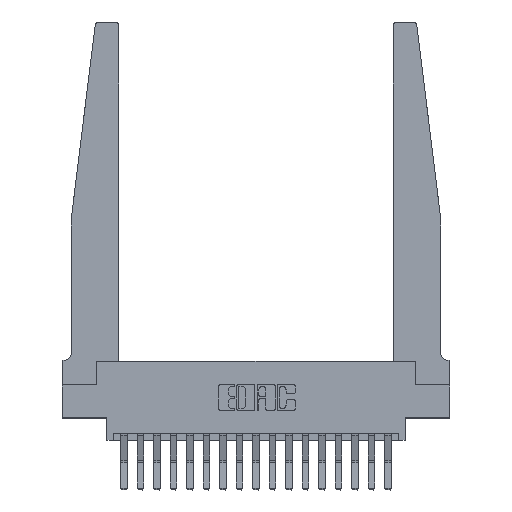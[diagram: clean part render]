
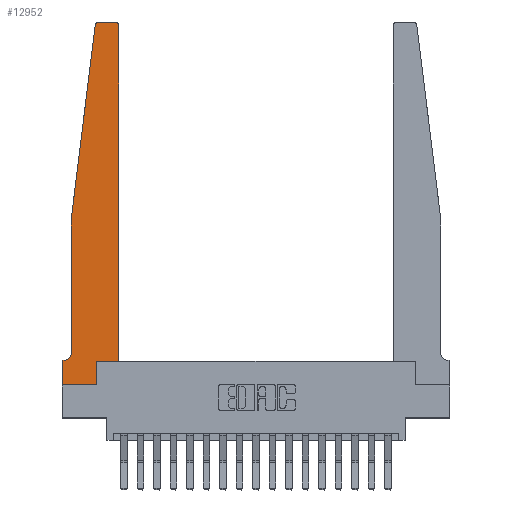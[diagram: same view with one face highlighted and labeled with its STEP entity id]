
A CAD part, top view. The second image highlights one B-rep face of the part: STEP entity #12952.
In plain terms, the highlighted planar face has unit normal (0, 0, 1).
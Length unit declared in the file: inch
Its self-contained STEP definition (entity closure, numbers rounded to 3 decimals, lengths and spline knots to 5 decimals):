
#132 = CARTESIAN_POINT ( 'NONE',  ( 0., 0.1875, 0.37 ) ) ;
#363 = VECTOR ( 'NONE', #8757, 39.37008 ) ;
#395 = VECTOR ( 'NONE', #5846, 39.37008 ) ;
#454 = CARTESIAN_POINT ( 'NONE',  ( 0.2605, 0., 0.37 ) ) ;
#477 = PLANE ( 'NONE',  #17138 ) ;
#569 = CARTESIAN_POINT ( 'NONE',  ( 0.24675, 2.72367, 0.37 ) ) ;
#772 = EDGE_CURVE ( 'NONE', #9024, #2285, #6179, .T. ) ;
#812 = ORIENTED_EDGE ( 'NONE', *, *, #9415, .T. ) ;
#907 = CARTESIAN_POINT ( 'NONE',  ( 0.395, 2.75, 0.37 ) ) ;
#1017 = EDGE_CURVE ( 'NONE', #3345, #19873, #10927, .T. ) ;
#1134 = ORIENTED_EDGE ( 'NONE', *, *, #4378, .T. ) ;
#1855 = CIRCLE ( 'NONE', #8939, 0.03 ) ;
#1858 = CARTESIAN_POINT ( 'NONE',  ( 0., 0., 0.37 ) ) ;
#1948 = VECTOR ( 'NONE', #12959, 39.37008 ) ;
#2080 = ORIENTED_EDGE ( 'NONE', *, *, #12305, .T. ) ;
#2121 = DIRECTION ( 'NONE',  ( -1., 0., 0. ) ) ;
#2285 = VERTEX_POINT ( 'NONE', #8772 ) ;
#2333 = VECTOR ( 'NONE', #6653, 39.37008 ) ;
#2542 = CARTESIAN_POINT ( 'NONE',  ( 0.425, 0.18, 0.37 ) ) ;
#3279 = VERTEX_POINT ( 'NONE', #5874 ) ;
#3345 = VERTEX_POINT ( 'NONE', #907 ) ;
#3388 = CARTESIAN_POINT ( 'NONE',  ( 0.425, 0.18, 0.37 ) ) ;
#3625 = CARTESIAN_POINT ( 'NONE',  ( 0.015, 0.2375, 0.37 ) ) ;
#3632 = EDGE_CURVE ( 'NONE', #3279, #8350, #10799, .T. ) ;
#3670 = LINE ( 'NONE', #9833, #16539 ) ;
#3738 = CIRCLE ( 'NONE', #11496, 0.03 ) ;
#3745 = VERTEX_POINT ( 'NONE', #15587 ) ;
#3759 = DIRECTION ( 'NONE',  ( -0.122, -0.992, 0. ) ) ;
#3786 = CARTESIAN_POINT ( 'NONE',  ( 0.27653, 2.72, 0.37 ) ) ;
#3845 = EDGE_CURVE ( 'NONE', #19873, #18053, #3738, .T. ) ;
#4378 = EDGE_CURVE ( 'NONE', #2285, #3745, #19816, .T. ) ;
#4546 = ORIENTED_EDGE ( 'NONE', *, *, #14837, .T. ) ;
#4710 = DIRECTION ( 'NONE',  ( 0., 0., 1. ) ) ;
#5146 = EDGE_CURVE ( 'NONE', #10796, #3345, #1855, .T. ) ;
#5281 = CARTESIAN_POINT ( 'NONE',  ( 0.395, 2.72, 0.37 ) ) ;
#5485 = DIRECTION ( 'NONE',  ( 1., 0., 0. ) ) ;
#5495 = CARTESIAN_POINT ( 'NONE',  ( 0.425, 2.72, 0.37 ) ) ;
#5846 = DIRECTION ( 'NONE',  ( 0., 1., 0. ) ) ;
#5874 = CARTESIAN_POINT ( 'NONE',  ( 0., 0., 0.37 ) ) ;
#5977 = DIRECTION ( 'NONE',  ( 0., -1., 0. ) ) ;
#6179 = LINE ( 'NONE', #16731, #19695 ) ;
#6653 = DIRECTION ( 'NONE',  ( -1., 0., 0. ) ) ;
#7195 = CARTESIAN_POINT ( 'NONE',  ( 0.27653, 2.75, 0.37 ) ) ;
#7223 = VECTOR ( 'NONE', #8010, 39.37008 ) ;
#8010 = DIRECTION ( 'NONE',  ( 0., -1., 0. ) ) ;
#8079 = DIRECTION ( 'NONE',  ( -1., 0., 0. ) ) ;
#8350 = VERTEX_POINT ( 'NONE', #454 ) ;
#8459 = EDGE_CURVE ( 'NONE', #11095, #10796, #19153, .T. ) ;
#8757 = DIRECTION ( 'NONE',  ( 1., 0., 0. ) ) ;
#8772 = CARTESIAN_POINT ( 'NONE',  ( 0.065, 0.2375, 0.37 ) ) ;
#8789 = VERTEX_POINT ( 'NONE', #132 ) ;
#8939 = AXIS2_PLACEMENT_3D ( 'NONE', #5281, #14077, #11458 ) ;
#8941 = VECTOR ( 'NONE', #19797, 39.37008 ) ;
#8980 = CARTESIAN_POINT ( 'NONE',  ( 0.065, 1.25, 0.37 ) ) ;
#9024 = VERTEX_POINT ( 'NONE', #8980 ) ;
#9089 = LINE ( 'NONE', #18223, #395 ) ;
#9396 = ORIENTED_EDGE ( 'NONE', *, *, #3632, .T. ) ;
#9415 = EDGE_CURVE ( 'NONE', #10102, #11095, #18305, .T. ) ;
#9480 = CARTESIAN_POINT ( 'NONE',  ( 0.065, 0.1875, 0.37 ) ) ;
#9833 = CARTESIAN_POINT ( 'NONE',  ( 0.065, 1.25, 0.37 ) ) ;
#10102 = VERTEX_POINT ( 'NONE', #13637 ) ;
#10314 = ORIENTED_EDGE ( 'NONE', *, *, #1017, .T. ) ;
#10402 = ORIENTED_EDGE ( 'NONE', *, *, #14713, .T. ) ;
#10688 = CARTESIAN_POINT ( 'NONE',  ( 0., 0., 0.37 ) ) ;
#10699 = CARTESIAN_POINT ( 'NONE',  ( 0.425, 0.18, 0.37 ) ) ;
#10796 = VERTEX_POINT ( 'NONE', #5495 ) ;
#10799 = LINE ( 'NONE', #10688, #8941 ) ;
#10888 = FACE_OUTER_BOUND ( 'NONE', #17705, .T. ) ;
#10927 = LINE ( 'NONE', #17325, #15064 ) ;
#11095 = VERTEX_POINT ( 'NONE', #3388 ) ;
#11170 = ORIENTED_EDGE ( 'NONE', *, *, #5146, .T. ) ;
#11389 = DIRECTION ( 'NONE',  ( 0., 0., 1. ) ) ;
#11458 = DIRECTION ( 'NONE',  ( 1., 0., 0. ) ) ;
#11496 = AXIS2_PLACEMENT_3D ( 'NONE', #3786, #11389, #5485 ) ;
#11811 = AXIS2_PLACEMENT_3D ( 'NONE', #3625, #15915, #2121 ) ;
#12305 = EDGE_CURVE ( 'NONE', #8350, #10102, #9089, .T. ) ;
#12462 = EDGE_CURVE ( 'NONE', #3745, #8789, #12516, .T. ) ;
#12516 = LINE ( 'NONE', #9480, #2333 ) ;
#12952 = ADVANCED_FACE ( 'NONE', ( #10888 ), #477, .T. ) ;
#12959 = DIRECTION ( 'NONE',  ( 0., 1., 0. ) ) ;
#13637 = CARTESIAN_POINT ( 'NONE',  ( 0.2605, 0.18, 0.37 ) ) ;
#14077 = DIRECTION ( 'NONE',  ( 0., 0., 1. ) ) ;
#14340 = ORIENTED_EDGE ( 'NONE', *, *, #8459, .T. ) ;
#14713 = EDGE_CURVE ( 'NONE', #8789, #3279, #18673, .T. ) ;
#14837 = EDGE_CURVE ( 'NONE', #18053, #9024, #3670, .T. ) ;
#15064 = VECTOR ( 'NONE', #8079, 39.37008 ) ;
#15121 = ORIENTED_EDGE ( 'NONE', *, *, #12462, .T. ) ;
#15587 = CARTESIAN_POINT ( 'NONE',  ( 0.015, 0.1875, 0.37 ) ) ;
#15788 = DIRECTION ( 'NONE',  ( 1., 0., 0. ) ) ;
#15915 = DIRECTION ( 'NONE',  ( 0., 0., -1. ) ) ;
#16340 = ORIENTED_EDGE ( 'NONE', *, *, #772, .T. ) ;
#16539 = VECTOR ( 'NONE', #3759, 39.37008 ) ;
#16636 = ORIENTED_EDGE ( 'NONE', *, *, #3845, .T. ) ;
#16731 = CARTESIAN_POINT ( 'NONE',  ( 0.065, 1.25, 0.37 ) ) ;
#17138 = AXIS2_PLACEMENT_3D ( 'NONE', #18697, #4710, #15788 ) ;
#17325 = CARTESIAN_POINT ( 'NONE',  ( 0.25, 2.75, 0.37 ) ) ;
#17705 = EDGE_LOOP ( 'NONE', ( #10314, #16636, #4546, #16340, #1134, #15121, #10402, #9396, #2080, #812, #14340, #11170 ) ) ;
#18053 = VERTEX_POINT ( 'NONE', #569 ) ;
#18223 = CARTESIAN_POINT ( 'NONE',  ( 0.2605, 0.18, 0.37 ) ) ;
#18305 = LINE ( 'NONE', #10699, #363 ) ;
#18673 = LINE ( 'NONE', #1858, #7223 ) ;
#18697 = CARTESIAN_POINT ( 'NONE',  ( 0., 0.1875, 0.37 ) ) ;
#19153 = LINE ( 'NONE', #2542, #1948 ) ;
#19695 = VECTOR ( 'NONE', #5977, 39.37008 ) ;
#19797 = DIRECTION ( 'NONE',  ( 1., 0., 0. ) ) ;
#19816 = CIRCLE ( 'NONE', #11811, 0.05 ) ;
#19873 = VERTEX_POINT ( 'NONE', #7195 ) ;
